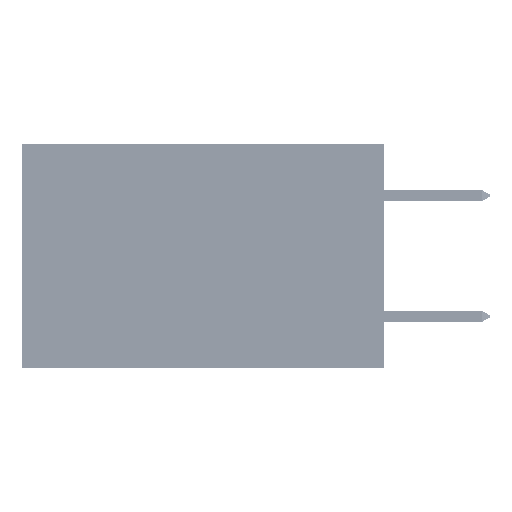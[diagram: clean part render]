
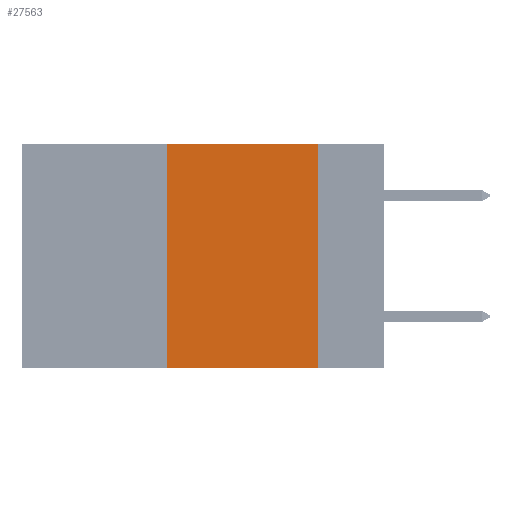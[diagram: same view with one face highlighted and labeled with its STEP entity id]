
A CAD part, left-side view. The second image highlights one B-rep face of the part: STEP entity #27563.
In plain terms, the highlighted planar face has unit normal (-1, 0, 0).
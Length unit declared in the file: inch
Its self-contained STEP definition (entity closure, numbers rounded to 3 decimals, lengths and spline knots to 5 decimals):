
#2671 = CARTESIAN_POINT ( 'NONE',  ( 0., 0.36, -0.37 ) ) ;
#3795 = DIRECTION ( 'NONE',  ( 0., 0., -1. ) ) ;
#4761 = FACE_OUTER_BOUND ( 'NONE', #31332, .T. ) ;
#4833 = VERTEX_POINT ( 'NONE', #34337 ) ;
#5318 = VERTEX_POINT ( 'NONE', #29037 ) ;
#7922 = VECTOR ( 'NONE', #26701, 39.37008 ) ;
#8576 = VECTOR ( 'NONE', #31471, 39.37008 ) ;
#10634 = VECTOR ( 'NONE', #13767, 39.37008 ) ;
#11887 = CARTESIAN_POINT ( 'NONE',  ( 0., 0.6, 0. ) ) ;
#13767 = DIRECTION ( 'NONE',  ( 0., -1., 0. ) ) ;
#14253 = ORIENTED_EDGE ( 'NONE', *, *, #32300, .F. ) ;
#14943 = CARTESIAN_POINT ( 'NONE',  ( 0., 0.6, -0.37 ) ) ;
#15433 = LINE ( 'NONE', #16982, #32150 ) ;
#16982 = CARTESIAN_POINT ( 'NONE',  ( 0., 0.11, 0. ) ) ;
#19515 = LINE ( 'NONE', #14943, #8576 ) ;
#21134 = DIRECTION ( 'NONE',  ( 0., 0., -1. ) ) ;
#22622 = CARTESIAN_POINT ( 'NONE',  ( 0., 0.36, 0. ) ) ;
#22625 = EDGE_CURVE ( 'NONE', #26008, #5318, #19515, .T. ) ;
#24271 = PLANE ( 'NONE',  #42417 ) ;
#26008 = VERTEX_POINT ( 'NONE', #2671 ) ;
#26701 = DIRECTION ( 'NONE',  ( 0., 0., 1. ) ) ;
#27563 = ADVANCED_FACE ( 'NONE', ( #4761 ), #24271, .F. ) ;
#28316 = CARTESIAN_POINT ( 'NONE',  ( 0., 0.36, 0. ) ) ;
#28395 = DIRECTION ( 'NONE',  ( 1., 0., 0. ) ) ;
#29037 = CARTESIAN_POINT ( 'NONE',  ( 0., 0.11, -0.37 ) ) ;
#30297 = CARTESIAN_POINT ( 'NONE',  ( 0., 0.6, 0. ) ) ;
#30857 = EDGE_CURVE ( 'NONE', #32561, #4833, #32520, .T. ) ;
#31020 = ORIENTED_EDGE ( 'NONE', *, *, #22625, .T. ) ;
#31063 = LINE ( 'NONE', #22622, #7922 ) ;
#31332 = EDGE_LOOP ( 'NONE', ( #49720, #32984, #14253, #31020 ) ) ;
#31471 = DIRECTION ( 'NONE',  ( 0., -1., 0. ) ) ;
#32150 = VECTOR ( 'NONE', #21134, 39.37008 ) ;
#32300 = EDGE_CURVE ( 'NONE', #26008, #32561, #31063, .T. ) ;
#32520 = LINE ( 'NONE', #30297, #10634 ) ;
#32561 = VERTEX_POINT ( 'NONE', #28316 ) ;
#32984 = ORIENTED_EDGE ( 'NONE', *, *, #30857, .F. ) ;
#34337 = CARTESIAN_POINT ( 'NONE',  ( 0., 0.11, 0. ) ) ;
#42417 = AXIS2_PLACEMENT_3D ( 'NONE', #11887, #28395, #3795 ) ;
#47045 = EDGE_CURVE ( 'NONE', #4833, #5318, #15433, .T. ) ;
#49720 = ORIENTED_EDGE ( 'NONE', *, *, #47045, .F. ) ;
